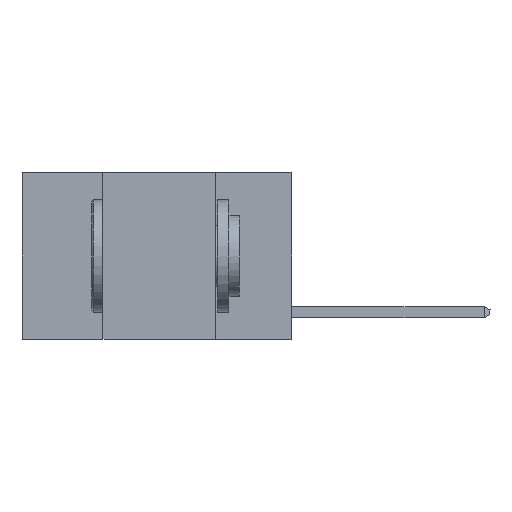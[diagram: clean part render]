
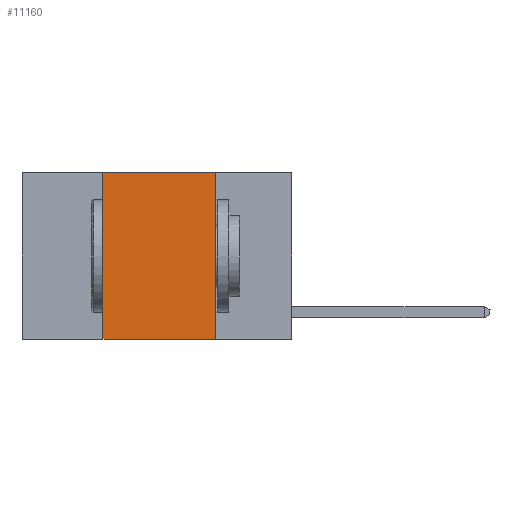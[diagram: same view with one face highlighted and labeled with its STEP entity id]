
A CAD part, left-side view. The second image highlights one B-rep face of the part: STEP entity #11160.
In plain terms, the highlighted planar face has unit normal (-1, 0, 0).
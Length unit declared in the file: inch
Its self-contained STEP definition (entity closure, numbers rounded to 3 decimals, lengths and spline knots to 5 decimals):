
#82 = VECTOR ( 'NONE', #8880, 39.37008 ) ;
#118 = VECTOR ( 'NONE', #8599, 39.37008 ) ;
#2078 = EDGE_LOOP ( 'NONE', ( #9511, #3393, #12658, #3813 ) ) ;
#2450 = DIRECTION ( 'NONE',  ( 1., 0., 0. ) ) ;
#2525 = CARTESIAN_POINT ( 'NONE',  ( 0., 0.6, -0.37 ) ) ;
#3393 = ORIENTED_EDGE ( 'NONE', *, *, #4466, .F. ) ;
#3512 = CARTESIAN_POINT ( 'NONE',  ( 0., 0.17, 0. ) ) ;
#3535 = VERTEX_POINT ( 'NONE', #8942 ) ;
#3537 = EDGE_CURVE ( 'NONE', #3535, #3805, #9682, .T. ) ;
#3541 = CARTESIAN_POINT ( 'NONE',  ( 0., 0.42, 0. ) ) ;
#3545 = LINE ( 'NONE', #7825, #4759 ) ;
#3805 = VERTEX_POINT ( 'NONE', #5475 ) ;
#3813 = ORIENTED_EDGE ( 'NONE', *, *, #10492, .T. ) ;
#4466 = EDGE_CURVE ( 'NONE', #3805, #5987, #9108, .T. ) ;
#4759 = VECTOR ( 'NONE', #10522, 39.37008 ) ;
#5475 = CARTESIAN_POINT ( 'NONE',  ( 0., 0.42, 0. ) ) ;
#5913 = CARTESIAN_POINT ( 'NONE',  ( 0., 0.6, 0. ) ) ;
#5987 = VERTEX_POINT ( 'NONE', #3512 ) ;
#7163 = CARTESIAN_POINT ( 'NONE',  ( 0., 0.17, -0.37 ) ) ;
#7790 = DIRECTION ( 'NONE',  ( 0., -1., 0. ) ) ;
#7825 = CARTESIAN_POINT ( 'NONE',  ( 0., 0.17, 0. ) ) ;
#7945 = CARTESIAN_POINT ( 'NONE',  ( 0., 0.6, 0. ) ) ;
#8599 = DIRECTION ( 'NONE',  ( 0., -1., 0. ) ) ;
#8604 = LINE ( 'NONE', #2525, #10291 ) ;
#8880 = DIRECTION ( 'NONE',  ( 0., 0., 1. ) ) ;
#8942 = CARTESIAN_POINT ( 'NONE',  ( 0., 0.42, -0.37 ) ) ;
#9108 = LINE ( 'NONE', #5913, #118 ) ;
#9511 = ORIENTED_EDGE ( 'NONE', *, *, #12483, .F. ) ;
#9682 = LINE ( 'NONE', #3541, #82 ) ;
#9690 = VERTEX_POINT ( 'NONE', #7163 ) ;
#10291 = VECTOR ( 'NONE', #7790, 39.37008 ) ;
#10492 = EDGE_CURVE ( 'NONE', #3535, #9690, #8604, .T. ) ;
#10522 = DIRECTION ( 'NONE',  ( 0., 0., -1. ) ) ;
#11160 = ADVANCED_FACE ( 'NONE', ( #15366 ), #13306, .F. ) ;
#12483 = EDGE_CURVE ( 'NONE', #5987, #9690, #3545, .T. ) ;
#12658 = ORIENTED_EDGE ( 'NONE', *, *, #3537, .F. ) ;
#13306 = PLANE ( 'NONE',  #14151 ) ;
#14151 = AXIS2_PLACEMENT_3D ( 'NONE', #7945, #2450, #15647 ) ;
#15366 = FACE_OUTER_BOUND ( 'NONE', #2078, .T. ) ;
#15647 = DIRECTION ( 'NONE',  ( 0., 0., -1. ) ) ;
